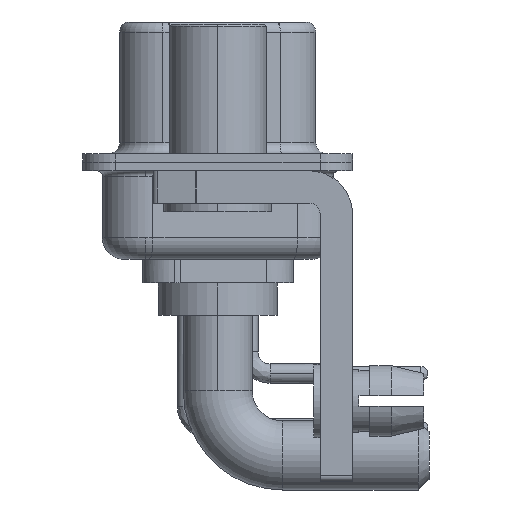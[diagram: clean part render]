
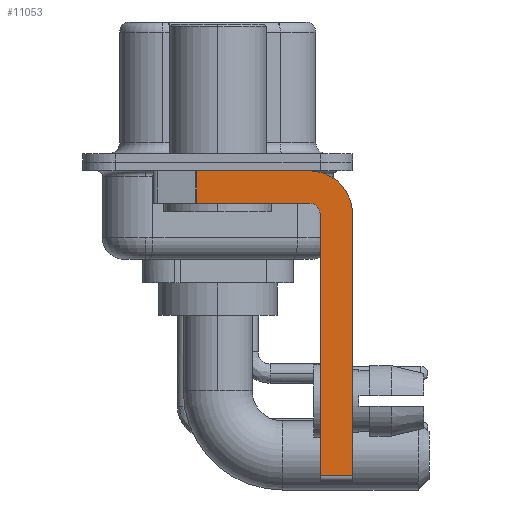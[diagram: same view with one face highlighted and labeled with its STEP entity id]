
A CAD part, left-side view. The second image highlights one B-rep face of the part: STEP entity #11053.
In plain terms, the highlighted planar face has unit normal (-1, 0, 0).
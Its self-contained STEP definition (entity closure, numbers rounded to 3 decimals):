
#34 = CARTESIAN_POINT ( 'NONE',  ( -2.9, -4.25, -14.55 ) ) ;
#100 = CARTESIAN_POINT ( 'NONE',  ( -2.9, -4.25, -2.4 ) ) ;
#204 = CARTESIAN_POINT ( 'NONE',  ( -2.9, -6.25, -2.4 ) ) ;
#442 = VECTOR ( 'NONE', #23729, 1000. ) ;
#1060 = ORIENTED_EDGE ( 'NONE', *, *, #20620, .F. ) ;
#1226 = CARTESIAN_POINT ( 'NONE',  ( -2.9, -4.25, -2.4 ) ) ;
#2103 = EDGE_CURVE ( 'NONE', #2106, #6060, #23304, .T. ) ;
#2106 = VERTEX_POINT ( 'NONE', #27975 ) ;
#2580 = ORIENTED_EDGE ( 'NONE', *, *, #17216, .T. ) ;
#2586 = CARTESIAN_POINT ( 'NONE',  ( -2.9, -4.75, -14.55 ) ) ;
#2907 = DIRECTION ( 'NONE',  ( 0., 1., 0. ) ) ;
#2942 = CARTESIAN_POINT ( 'NONE',  ( -2.9, -4.75, -14.8 ) ) ;
#2972 = CARTESIAN_POINT ( 'NONE',  ( -2.9, -4.25, -1.9 ) ) ;
#3259 = VERTEX_POINT ( 'NONE', #4958 ) ;
#3909 = EDGE_LOOP ( 'NONE', ( #6392, #2580, #1060, #12081, #8385, #18933, #21544, #6191 ) ) ;
#4274 = EDGE_CURVE ( 'NONE', #3259, #23892, #19638, .T. ) ;
#4658 = VECTOR ( 'NONE', #2907, 1000. ) ;
#4958 = CARTESIAN_POINT ( 'NONE',  ( -2.9, -6.25, -2.4 ) ) ;
#6007 = CARTESIAN_POINT ( 'NONE',  ( -2.9, 3., -0.4 ) ) ;
#6060 = VERTEX_POINT ( 'NONE', #9756 ) ;
#6134 = CARTESIAN_POINT ( 'NONE',  ( -2.9, 0.978, -1.9 ) ) ;
#6191 = ORIENTED_EDGE ( 'NONE', *, *, #26176, .F. ) ;
#6267 = EDGE_CURVE ( 'NONE', #10046, #16928, #13434, .T. ) ;
#6273 = VECTOR ( 'NONE', #8683, 1000. ) ;
#6392 = ORIENTED_EDGE ( 'NONE', *, *, #2103, .F. ) ;
#6579 = VERTEX_POINT ( 'NONE', #6134 ) ;
#7035 = LINE ( 'NONE', #17954, #4658 ) ;
#8210 = DIRECTION ( 'NONE',  ( 0., 0., -1. ) ) ;
#8385 = ORIENTED_EDGE ( 'NONE', *, *, #6267, .F. ) ;
#8536 = CARTESIAN_POINT ( 'NONE',  ( -2.9, -6.25, -14.55 ) ) ;
#8683 = DIRECTION ( 'NONE',  ( 0., -1., 0. ) ) ;
#8858 = DIRECTION ( 'NONE',  ( 0., 0., -1. ) ) ;
#9074 = EDGE_CURVE ( 'NONE', #16928, #20255, #25946, .T. ) ;
#9756 = CARTESIAN_POINT ( 'NONE',  ( -2.9, -4.25, -0.4 ) ) ;
#10021 = FACE_OUTER_BOUND ( 'NONE', #3909, .T. ) ;
#10046 = VERTEX_POINT ( 'NONE', #2586 ) ;
#11053 = ADVANCED_FACE ( 'NONE', ( #10021 ), #11857, .F. ) ;
#11857 = PLANE ( 'NONE',  #17458 ) ;
#12081 = ORIENTED_EDGE ( 'NONE', *, *, #9074, .F. ) ;
#13434 = LINE ( 'NONE', #2942, #14542 ) ;
#14318 = AXIS2_PLACEMENT_3D ( 'NONE', #25131, #25279, #27541 ) ;
#14542 = VECTOR ( 'NONE', #26489, 1000. ) ;
#14904 = LINE ( 'NONE', #34, #6273 ) ;
#16867 = AXIS2_PLACEMENT_3D ( 'NONE', #100, #21939, #22080 ) ;
#16928 = VERTEX_POINT ( 'NONE', #22048 ) ;
#17216 = EDGE_CURVE ( 'NONE', #2106, #6579, #27766, .T. ) ;
#17286 = CARTESIAN_POINT ( 'NONE',  ( -2.9, 0.978, -1.9 ) ) ;
#17458 = AXIS2_PLACEMENT_3D ( 'NONE', #1226, #27176, #20509 ) ;
#17954 = CARTESIAN_POINT ( 'NONE',  ( -2.9, -4.25, -1.9 ) ) ;
#18933 = ORIENTED_EDGE ( 'NONE', *, *, #27625, .T. ) ;
#19638 = LINE ( 'NONE', #204, #24619 ) ;
#20255 = VERTEX_POINT ( 'NONE', #2972 ) ;
#20509 = DIRECTION ( 'NONE',  ( 0., 0., -1. ) ) ;
#20620 = EDGE_CURVE ( 'NONE', #20255, #6579, #7035, .T. ) ;
#21544 = ORIENTED_EDGE ( 'NONE', *, *, #4274, .F. ) ;
#21939 = DIRECTION ( 'NONE',  ( -1., 0., 0. ) ) ;
#22048 = CARTESIAN_POINT ( 'NONE',  ( -2.9, -4.75, -2.4 ) ) ;
#22080 = DIRECTION ( 'NONE',  ( 0., 0., 1. ) ) ;
#23304 = LINE ( 'NONE', #6007, #442 ) ;
#23729 = DIRECTION ( 'NONE',  ( 0., -1., 0. ) ) ;
#23871 = CIRCLE ( 'NONE', #14318, 2. ) ;
#23892 = VERTEX_POINT ( 'NONE', #8536 ) ;
#24440 = VECTOR ( 'NONE', #8210, 1000. ) ;
#24619 = VECTOR ( 'NONE', #8858, 1000. ) ;
#25131 = CARTESIAN_POINT ( 'NONE',  ( -2.9, -4.25, -2.4 ) ) ;
#25279 = DIRECTION ( 'NONE',  ( 1., 0., 0. ) ) ;
#25946 = CIRCLE ( 'NONE', #16867, 0.5 ) ;
#26176 = EDGE_CURVE ( 'NONE', #6060, #3259, #23871, .T. ) ;
#26489 = DIRECTION ( 'NONE',  ( 0., 0., 1. ) ) ;
#27176 = DIRECTION ( 'NONE',  ( 1., 0., 0. ) ) ;
#27541 = DIRECTION ( 'NONE',  ( 0., 0., -1. ) ) ;
#27625 = EDGE_CURVE ( 'NONE', #10046, #23892, #14904, .T. ) ;
#27766 = LINE ( 'NONE', #17286, #24440 ) ;
#27975 = CARTESIAN_POINT ( 'NONE',  ( -2.9, 0.978, -0.4 ) ) ;
